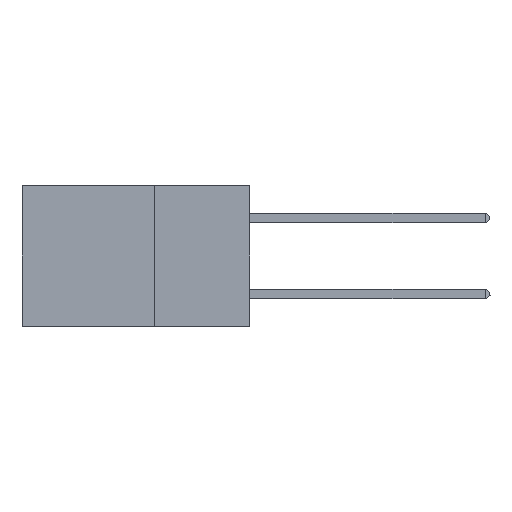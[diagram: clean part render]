
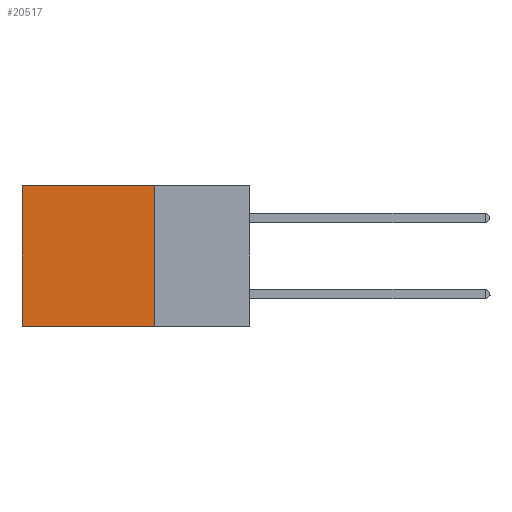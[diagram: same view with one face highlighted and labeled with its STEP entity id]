
A CAD part, left-side view. The second image highlights one B-rep face of the part: STEP entity #20517.
In plain terms, the highlighted planar face has unit normal (-1, 0, 0).
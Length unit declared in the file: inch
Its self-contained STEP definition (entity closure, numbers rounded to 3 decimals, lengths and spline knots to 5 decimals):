
#918 = EDGE_CURVE ( 'NONE', #21438, #7961, #22551, .T. ) ;
#1206 = CARTESIAN_POINT ( 'NONE',  ( 0.2875, 0.25, 0. ) ) ;
#1265 = DIRECTION ( 'NONE',  ( 0., 1., 0. ) ) ;
#2186 = CARTESIAN_POINT ( 'NONE',  ( 0.2875, 0.25, 0. ) ) ;
#2936 = ORIENTED_EDGE ( 'NONE', *, *, #3270, .F. ) ;
#3263 = VERTEX_POINT ( 'NONE', #5464 ) ;
#3270 = EDGE_CURVE ( 'NONE', #3263, #17598, #21366, .T. ) ;
#3855 = ORIENTED_EDGE ( 'NONE', *, *, #6103, .F. ) ;
#3951 = AXIS2_PLACEMENT_3D ( 'NONE', #18647, #12806, #16543 ) ;
#4948 = DIRECTION ( 'NONE',  ( 0., 0., -1. ) ) ;
#4976 = CARTESIAN_POINT ( 'NONE',  ( 0.2875, 0.6, 0. ) ) ;
#5291 = CARTESIAN_POINT ( 'NONE',  ( 0.2875, 0.25, -0.37 ) ) ;
#5464 = CARTESIAN_POINT ( 'NONE',  ( 0.2875, 0.25, -0.37 ) ) ;
#6103 = EDGE_CURVE ( 'NONE', #21438, #3263, #11167, .T. ) ;
#6187 = DIRECTION ( 'NONE',  ( 0., 1., 0. ) ) ;
#6263 = FACE_OUTER_BOUND ( 'NONE', #25310, .T. ) ;
#6454 = VECTOR ( 'NONE', #8787, 39.37008 ) ;
#6847 = PLANE ( 'NONE',  #3951 ) ;
#7019 = EDGE_CURVE ( 'NONE', #7961, #17598, #7385, .T. ) ;
#7385 = LINE ( 'NONE', #4976, #6454 ) ;
#7961 = VERTEX_POINT ( 'NONE', #18271 ) ;
#8787 = DIRECTION ( 'NONE',  ( 0., 0., -1. ) ) ;
#9906 = VECTOR ( 'NONE', #4948, 39.37008 ) ;
#10949 = ORIENTED_EDGE ( 'NONE', *, *, #7019, .T. ) ;
#11167 = LINE ( 'NONE', #1206, #9906 ) ;
#12806 = DIRECTION ( 'NONE',  ( 1., 0., 0. ) ) ;
#15226 = CARTESIAN_POINT ( 'NONE',  ( 0.2875, 0.6, -0.37 ) ) ;
#16543 = DIRECTION ( 'NONE',  ( 0., 0., -1. ) ) ;
#17598 = VERTEX_POINT ( 'NONE', #15226 ) ;
#17710 = ORIENTED_EDGE ( 'NONE', *, *, #918, .T. ) ;
#18271 = CARTESIAN_POINT ( 'NONE',  ( 0.2875, 0.6, 0. ) ) ;
#18647 = CARTESIAN_POINT ( 'NONE',  ( 0.2875, 0.25, 0. ) ) ;
#18775 = VECTOR ( 'NONE', #6187, 39.37008 ) ;
#18840 = VECTOR ( 'NONE', #1265, 39.37008 ) ;
#20517 = ADVANCED_FACE ( 'NONE', ( #6263 ), #6847, .F. ) ;
#21366 = LINE ( 'NONE', #5291, #18840 ) ;
#21438 = VERTEX_POINT ( 'NONE', #23138 ) ;
#22551 = LINE ( 'NONE', #2186, #18775 ) ;
#23138 = CARTESIAN_POINT ( 'NONE',  ( 0.2875, 0.25, 0. ) ) ;
#25310 = EDGE_LOOP ( 'NONE', ( #10949, #2936, #3855, #17710 ) ) ;
